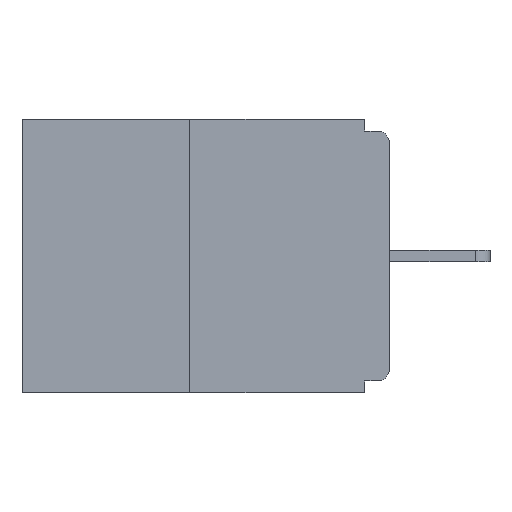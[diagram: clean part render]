
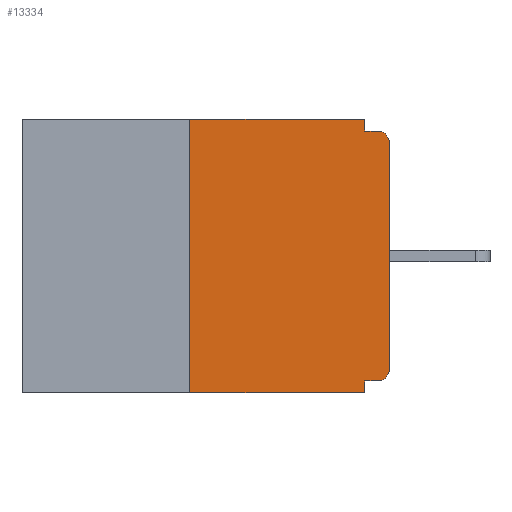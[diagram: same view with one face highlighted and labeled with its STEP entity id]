
A CAD part, left-side view. The second image highlights one B-rep face of the part: STEP entity #13334.
In plain terms, the highlighted planar face has unit normal (-1, 0, 0).
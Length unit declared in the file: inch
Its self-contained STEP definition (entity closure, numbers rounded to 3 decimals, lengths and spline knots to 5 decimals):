
#174 = VERTEX_POINT ( 'NONE', #4834 ) ;
#260 = DIRECTION ( 'NONE',  ( 0., 0., -1. ) ) ;
#390 = CARTESIAN_POINT ( 'NONE',  ( 0., 0.015, -0.03 ) ) ;
#613 = VERTEX_POINT ( 'NONE', #2848 ) ;
#678 = VERTEX_POINT ( 'NONE', #679 ) ;
#679 = CARTESIAN_POINT ( 'NONE',  ( 0., 0., -0.313 ) ) ;
#729 = CARTESIAN_POINT ( 'NONE',  ( 0., 0.015, -0.313 ) ) ;
#1070 = DIRECTION ( 'NONE',  ( 1., 0., 0. ) ) ;
#1093 = VECTOR ( 'NONE', #260, 39.37008 ) ;
#1542 = EDGE_CURVE ( 'NONE', #174, #6425, #9525, .T. ) ;
#2225 = DIRECTION ( 'NONE',  ( 0., 0., -1. ) ) ;
#2337 = DIRECTION ( 'NONE',  ( 0., -1., 0. ) ) ;
#2394 = FACE_OUTER_BOUND ( 'NONE', #5012, .T. ) ;
#2399 = EDGE_CURVE ( 'NONE', #613, #4606, #6579, .T. ) ;
#2785 = ORIENTED_EDGE ( 'NONE', *, *, #13415, .F. ) ;
#2833 = CARTESIAN_POINT ( 'NONE',  ( 0., 0.031, -0.328 ) ) ;
#2848 = CARTESIAN_POINT ( 'NONE',  ( 0., 0.25, 0. ) ) ;
#3246 = ORIENTED_EDGE ( 'NONE', *, *, #1542, .F. ) ;
#3468 = DIRECTION ( 'NONE',  ( 0., 0., -1. ) ) ;
#3486 = DIRECTION ( 'NONE',  ( -1., 0., 0. ) ) ;
#3487 = CARTESIAN_POINT ( 'NONE',  ( 0., 0., -0.03 ) ) ;
#3717 = ORIENTED_EDGE ( 'NONE', *, *, #16179, .T. ) ;
#3748 = VERTEX_POINT ( 'NONE', #10554 ) ;
#4343 = CARTESIAN_POINT ( 'NONE',  ( 0., 0., -0.015 ) ) ;
#4606 = VERTEX_POINT ( 'NONE', #12770 ) ;
#4652 = ORIENTED_EDGE ( 'NONE', *, *, #7969, .F. ) ;
#4834 = CARTESIAN_POINT ( 'NONE',  ( 0., 0.015, -0.328 ) ) ;
#5012 = EDGE_LOOP ( 'NONE', ( #13492, #2785, #6761, #18058, #3246, #3717, #11513, #15236, #8078, #4652 ) ) ;
#5363 = CARTESIAN_POINT ( 'NONE',  ( 0., 0.46, -0.343 ) ) ;
#5660 = VECTOR ( 'NONE', #11435, 39.37008 ) ;
#5745 = CARTESIAN_POINT ( 'NONE',  ( 0., 0.031, -0.343 ) ) ;
#5867 = VECTOR ( 'NONE', #8827, 39.37008 ) ;
#5997 = VERTEX_POINT ( 'NONE', #3487 ) ;
#6096 = VECTOR ( 'NONE', #2337, 39.37008 ) ;
#6425 = VERTEX_POINT ( 'NONE', #2833 ) ;
#6579 = LINE ( 'NONE', #17028, #6096 ) ;
#6641 = EDGE_CURVE ( 'NONE', #5997, #17363, #10064, .T. ) ;
#6661 = CARTESIAN_POINT ( 'NONE',  ( 0., 0.015, -0.015 ) ) ;
#6761 = ORIENTED_EDGE ( 'NONE', *, *, #7617, .T. ) ;
#7161 = CARTESIAN_POINT ( 'NONE',  ( 0., 0.25, 0. ) ) ;
#7617 = EDGE_CURVE ( 'NONE', #3748, #16775, #8450, .T. ) ;
#7658 = VECTOR ( 'NONE', #16024, 39.37008 ) ;
#7969 = EDGE_CURVE ( 'NONE', #4606, #9236, #12764, .T. ) ;
#8078 = ORIENTED_EDGE ( 'NONE', *, *, #10120, .F. ) ;
#8450 = LINE ( 'NONE', #5363, #18411 ) ;
#8827 = DIRECTION ( 'NONE',  ( 0., -1., 0. ) ) ;
#9236 = VERTEX_POINT ( 'NONE', #12249 ) ;
#9525 = LINE ( 'NONE', #11516, #5660 ) ;
#9851 = CARTESIAN_POINT ( 'NONE',  ( 0., 0.46, 0. ) ) ;
#10064 = CIRCLE ( 'NONE', #17448, 0.015 ) ;
#10120 = EDGE_CURVE ( 'NONE', #9236, #17363, #13992, .T. ) ;
#10554 = CARTESIAN_POINT ( 'NONE',  ( 0., 0.25, -0.343 ) ) ;
#10734 = CARTESIAN_POINT ( 'NONE',  ( 0., 0.031, 0. ) ) ;
#10994 = DIRECTION ( 'NONE',  ( -1., 0., 0. ) ) ;
#11005 = DIRECTION ( 'NONE',  ( 0., -1., 0. ) ) ;
#11336 = DIRECTION ( 'NONE',  ( 0., 0., -1. ) ) ;
#11435 = DIRECTION ( 'NONE',  ( 0., 1., 0. ) ) ;
#11513 = ORIENTED_EDGE ( 'NONE', *, *, #14770, .T. ) ;
#11516 = CARTESIAN_POINT ( 'NONE',  ( 0., 0., -0.328 ) ) ;
#11783 = VECTOR ( 'NONE', #14274, 39.37008 ) ;
#11811 = CARTESIAN_POINT ( 'NONE',  ( 0., 0., 0. ) ) ;
#12160 = CIRCLE ( 'NONE', #18031, 0.015 ) ;
#12238 = LINE ( 'NONE', #7161, #11783 ) ;
#12249 = CARTESIAN_POINT ( 'NONE',  ( 0., 0.031, -0.015 ) ) ;
#12374 = CARTESIAN_POINT ( 'NONE',  ( 0., 0.031, -0.343 ) ) ;
#12764 = LINE ( 'NONE', #10734, #1093 ) ;
#12770 = CARTESIAN_POINT ( 'NONE',  ( 0., 0.031, 0. ) ) ;
#12831 = EDGE_CURVE ( 'NONE', #6425, #16775, #14859, .T. ) ;
#13334 = ADVANCED_FACE ( 'NONE', ( #2394 ), #18286, .F. ) ;
#13415 = EDGE_CURVE ( 'NONE', #3748, #613, #12238, .T. ) ;
#13492 = ORIENTED_EDGE ( 'NONE', *, *, #2399, .F. ) ;
#13992 = LINE ( 'NONE', #4343, #5867 ) ;
#14274 = DIRECTION ( 'NONE',  ( 0., 0., 1. ) ) ;
#14350 = DIRECTION ( 'NONE',  ( 0., 0., -1. ) ) ;
#14370 = LINE ( 'NONE', #11811, #7658 ) ;
#14419 = VECTOR ( 'NONE', #14350, 39.37008 ) ;
#14770 = EDGE_CURVE ( 'NONE', #678, #5997, #14370, .T. ) ;
#14859 = LINE ( 'NONE', #5745, #14419 ) ;
#15236 = ORIENTED_EDGE ( 'NONE', *, *, #6641, .T. ) ;
#16024 = DIRECTION ( 'NONE',  ( 0., 0., 1. ) ) ;
#16179 = EDGE_CURVE ( 'NONE', #174, #678, #12160, .T. ) ;
#16775 = VERTEX_POINT ( 'NONE', #12374 ) ;
#16851 = AXIS2_PLACEMENT_3D ( 'NONE', #9851, #1070, #11336 ) ;
#17028 = CARTESIAN_POINT ( 'NONE',  ( 0., 0.46, 0. ) ) ;
#17363 = VERTEX_POINT ( 'NONE', #6661 ) ;
#17448 = AXIS2_PLACEMENT_3D ( 'NONE', #390, #3486, #3468 ) ;
#18031 = AXIS2_PLACEMENT_3D ( 'NONE', #729, #10994, #2225 ) ;
#18058 = ORIENTED_EDGE ( 'NONE', *, *, #12831, .F. ) ;
#18286 = PLANE ( 'NONE',  #16851 ) ;
#18411 = VECTOR ( 'NONE', #11005, 39.37008 ) ;
